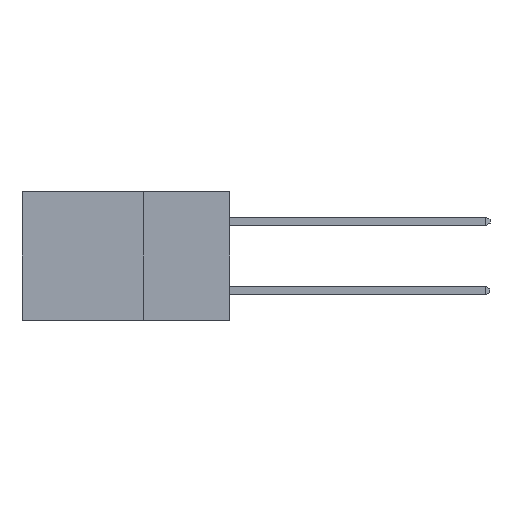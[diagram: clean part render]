
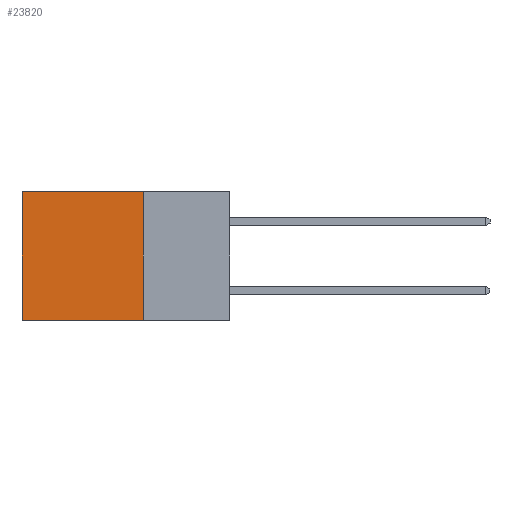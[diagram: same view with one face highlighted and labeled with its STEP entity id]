
A CAD part, left-side view. The second image highlights one B-rep face of the part: STEP entity #23820.
In plain terms, the highlighted planar face has unit normal (-1, 0, 0).
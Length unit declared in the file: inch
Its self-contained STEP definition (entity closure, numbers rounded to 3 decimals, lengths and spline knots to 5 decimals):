
#115 = CARTESIAN_POINT ( 'NONE',  ( 0.298, 0.25, 0. ) ) ;
#1833 = CARTESIAN_POINT ( 'NONE',  ( 0.298, 0.25, 0. ) ) ;
#2173 = DIRECTION ( 'NONE',  ( 0., 1., 0. ) ) ;
#2685 = LINE ( 'NONE', #18024, #12935 ) ;
#4092 = VERTEX_POINT ( 'NONE', #6796 ) ;
#4601 = FACE_OUTER_BOUND ( 'NONE', #18821, .T. ) ;
#4912 = EDGE_CURVE ( 'NONE', #6186, #16616, #5043, .T. ) ;
#5043 = LINE ( 'NONE', #11509, #20539 ) ;
#5199 = ORIENTED_EDGE ( 'NONE', *, *, #20694, .T. ) ;
#5733 = ORIENTED_EDGE ( 'NONE', *, *, #22412, .F. ) ;
#6186 = VERTEX_POINT ( 'NONE', #21381 ) ;
#6250 = ORIENTED_EDGE ( 'NONE', *, *, #4912, .F. ) ;
#6796 = CARTESIAN_POINT ( 'NONE',  ( 0.298, 0.25, 0. ) ) ;
#9936 = DIRECTION ( 'NONE',  ( 1., 0., 0. ) ) ;
#10919 = ORIENTED_EDGE ( 'NONE', *, *, #16023, .T. ) ;
#11454 = LINE ( 'NONE', #1833, #21422 ) ;
#11509 = CARTESIAN_POINT ( 'NONE',  ( 0.298, 0.25, -0.37 ) ) ;
#11862 = CARTESIAN_POINT ( 'NONE',  ( 0.298, 0.6, -0.37 ) ) ;
#12935 = VECTOR ( 'NONE', #16091, 39.37008 ) ;
#13506 = DIRECTION ( 'NONE',  ( 0., 1., 0. ) ) ;
#14074 = DIRECTION ( 'NONE',  ( 0., 0., -1. ) ) ;
#15876 = LINE ( 'NONE', #115, #25836 ) ;
#16023 = EDGE_CURVE ( 'NONE', #20348, #16616, #2685, .T. ) ;
#16091 = DIRECTION ( 'NONE',  ( 0., 0., -1. ) ) ;
#16374 = AXIS2_PLACEMENT_3D ( 'NONE', #17909, #9936, #23881 ) ;
#16616 = VERTEX_POINT ( 'NONE', #11862 ) ;
#17909 = CARTESIAN_POINT ( 'NONE',  ( 0.298, 0.25, 0. ) ) ;
#18024 = CARTESIAN_POINT ( 'NONE',  ( 0.298, 0.6, 0. ) ) ;
#18821 = EDGE_LOOP ( 'NONE', ( #10919, #6250, #5733, #5199 ) ) ;
#19412 = CARTESIAN_POINT ( 'NONE',  ( 0.298, 0.6, 0. ) ) ;
#20348 = VERTEX_POINT ( 'NONE', #19412 ) ;
#20539 = VECTOR ( 'NONE', #13506, 39.37008 ) ;
#20694 = EDGE_CURVE ( 'NONE', #4092, #20348, #15876, .T. ) ;
#21381 = CARTESIAN_POINT ( 'NONE',  ( 0.298, 0.25, -0.37 ) ) ;
#21422 = VECTOR ( 'NONE', #14074, 39.37008 ) ;
#21876 = PLANE ( 'NONE',  #16374 ) ;
#22412 = EDGE_CURVE ( 'NONE', #4092, #6186, #11454, .T. ) ;
#23820 = ADVANCED_FACE ( 'NONE', ( #4601 ), #21876, .F. ) ;
#23881 = DIRECTION ( 'NONE',  ( 0., 0., -1. ) ) ;
#25836 = VECTOR ( 'NONE', #2173, 39.37008 ) ;
